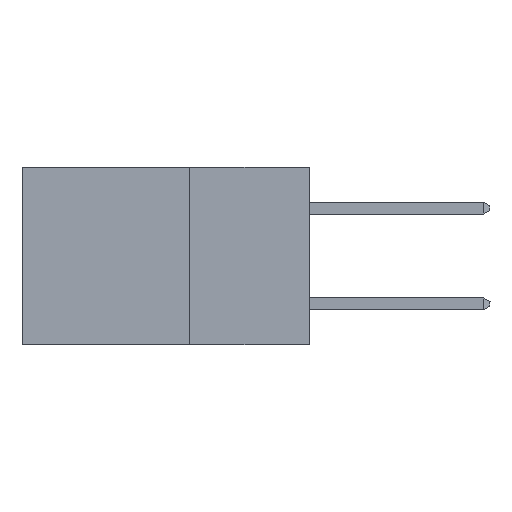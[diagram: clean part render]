
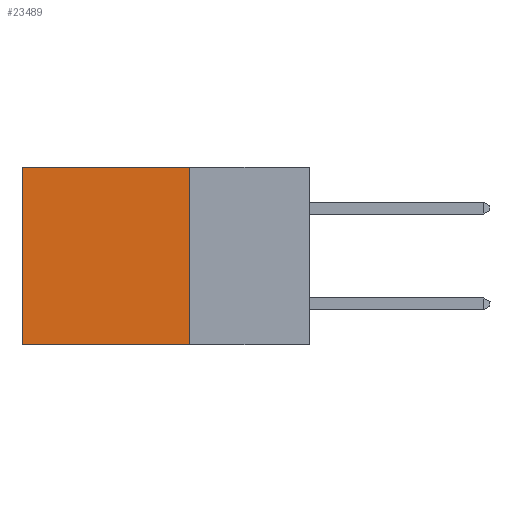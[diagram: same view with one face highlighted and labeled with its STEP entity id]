
A CAD part, left-side view. The second image highlights one B-rep face of the part: STEP entity #23489.
In plain terms, the highlighted planar face has unit normal (-1, 0, 0).
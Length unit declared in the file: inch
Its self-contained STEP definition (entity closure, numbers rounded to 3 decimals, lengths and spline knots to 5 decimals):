
#752 = VERTEX_POINT ( 'NONE', #22999 ) ;
#1214 = CARTESIAN_POINT ( 'NONE',  ( 0.2875, 0.6, 0. ) ) ;
#1385 = CARTESIAN_POINT ( 'NONE',  ( 0.2875, 0.25, 0. ) ) ;
#2604 = DIRECTION ( 'NONE',  ( 0., 1., 0. ) ) ;
#3776 = CARTESIAN_POINT ( 'NONE',  ( 0.2875, 0.25, 0. ) ) ;
#4036 = VERTEX_POINT ( 'NONE', #32942 ) ;
#4311 = ORIENTED_EDGE ( 'NONE', *, *, #28546, .F. ) ;
#4546 = VECTOR ( 'NONE', #14081, 39.37008 ) ;
#4685 = EDGE_CURVE ( 'NONE', #33278, #25202, #38147, .T. ) ;
#6207 = ORIENTED_EDGE ( 'NONE', *, *, #37786, .F. ) ;
#6918 = EDGE_CURVE ( 'NONE', #25202, #752, #19763, .T. ) ;
#11054 = VECTOR ( 'NONE', #33080, 39.37008 ) ;
#13423 = EDGE_LOOP ( 'NONE', ( #15551, #6207, #4311, #35674 ) ) ;
#13741 = VECTOR ( 'NONE', #38469, 39.37008 ) ;
#14081 = DIRECTION ( 'NONE',  ( 0., 1., 0. ) ) ;
#15551 = ORIENTED_EDGE ( 'NONE', *, *, #6918, .T. ) ;
#15709 = CARTESIAN_POINT ( 'NONE',  ( 0.2875, 0.25, 0. ) ) ;
#19763 = LINE ( 'NONE', #1214, #11054 ) ;
#20454 = DIRECTION ( 'NONE',  ( 0., 0., -1. ) ) ;
#22999 = CARTESIAN_POINT ( 'NONE',  ( 0.2875, 0.6, -0.37 ) ) ;
#23489 = ADVANCED_FACE ( 'NONE', ( #26966 ), #40324, .F. ) ;
#24189 = DIRECTION ( 'NONE',  ( 1., 0., 0. ) ) ;
#25202 = VERTEX_POINT ( 'NONE', #39723 ) ;
#26966 = FACE_OUTER_BOUND ( 'NONE', #13423, .T. ) ;
#28439 = LINE ( 'NONE', #28592, #36996 ) ;
#28546 = EDGE_CURVE ( 'NONE', #33278, #4036, #31111, .T. ) ;
#28592 = CARTESIAN_POINT ( 'NONE',  ( 0.2875, 0.25, -0.37 ) ) ;
#29286 = AXIS2_PLACEMENT_3D ( 'NONE', #1385, #24189, #20454 ) ;
#31111 = LINE ( 'NONE', #15709, #13741 ) ;
#32942 = CARTESIAN_POINT ( 'NONE',  ( 0.2875, 0.25, -0.37 ) ) ;
#33080 = DIRECTION ( 'NONE',  ( 0., 0., -1. ) ) ;
#33278 = VERTEX_POINT ( 'NONE', #3776 ) ;
#33895 = CARTESIAN_POINT ( 'NONE',  ( 0.2875, 0.25, 0. ) ) ;
#35674 = ORIENTED_EDGE ( 'NONE', *, *, #4685, .T. ) ;
#36996 = VECTOR ( 'NONE', #2604, 39.37008 ) ;
#37786 = EDGE_CURVE ( 'NONE', #4036, #752, #28439, .T. ) ;
#38147 = LINE ( 'NONE', #33895, #4546 ) ;
#38469 = DIRECTION ( 'NONE',  ( 0., 0., -1. ) ) ;
#39723 = CARTESIAN_POINT ( 'NONE',  ( 0.2875, 0.6, 0. ) ) ;
#40324 = PLANE ( 'NONE',  #29286 ) ;
